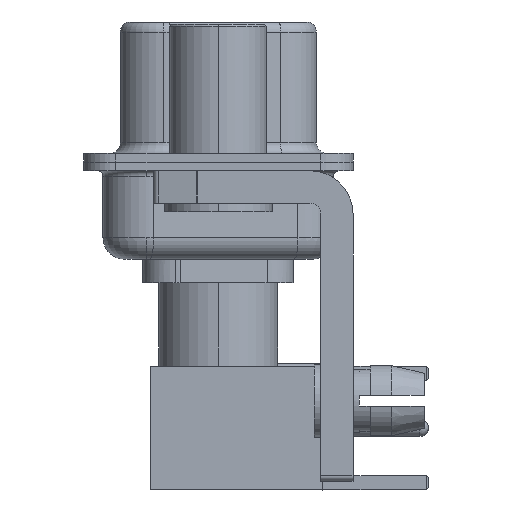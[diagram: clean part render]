
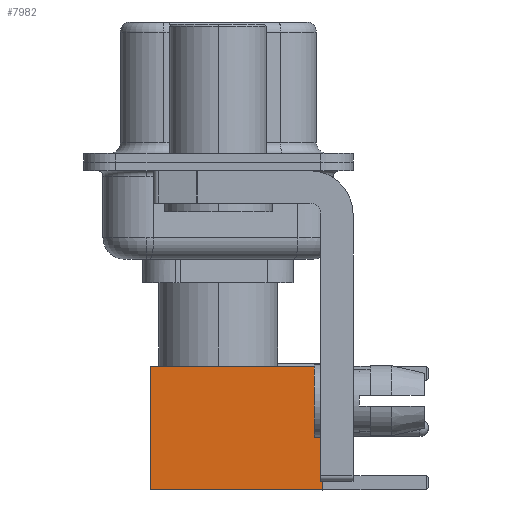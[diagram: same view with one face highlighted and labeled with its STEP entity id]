
A CAD part, left-side view. The second image highlights one B-rep face of the part: STEP entity #7982.
In plain terms, the highlighted face is planar.
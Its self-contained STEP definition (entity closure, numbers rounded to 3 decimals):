
#1560 = ORIENTED_EDGE ( 'NONE', *, *, #9778, .T. ) ;
#3294 = EDGE_CURVE ( 'NONE', #36083, #10672, #4469, .T. ) ;
#3545 = ORIENTED_EDGE ( 'NONE', *, *, #3294, .T. ) ;
#4402 = DIRECTION ( 'NONE',  ( 0., 0., -1. ) ) ;
#4469 = LINE ( 'NONE', #32501, #7651 ) ;
#4936 = VECTOR ( 'NONE', #4402, 1000. ) ;
#7360 = CARTESIAN_POINT ( 'NONE',  ( 2.875, 2.875, 0. ) ) ;
#7651 = VECTOR ( 'NONE', #9873, 1000. ) ;
#7982 = ADVANCED_FACE ( 'NONE', ( #8648 ), #34427, .T. ) ;
#8456 = AXIS2_PLACEMENT_3D ( 'NONE', #28863, #31286, #8818 ) ;
#8648 = FACE_OUTER_BOUND ( 'NONE', #25644, .T. ) ;
#8818 = DIRECTION ( 'NONE',  ( 0., 0., 1. ) ) ;
#9072 = DIRECTION ( 'NONE',  ( -1., 0., 0. ) ) ;
#9778 = EDGE_CURVE ( 'NONE', #26806, #36083, #9988, .T. ) ;
#9873 = DIRECTION ( 'NONE',  ( -1., 0., 0. ) ) ;
#9988 = LINE ( 'NONE', #16108, #4936 ) ;
#10267 = VECTOR ( 'NONE', #9072, 1000. ) ;
#10672 = VERTEX_POINT ( 'NONE', #14701 ) ;
#11019 = CARTESIAN_POINT ( 'NONE',  ( -2.875, 2.875, 8. ) ) ;
#11522 = LINE ( 'NONE', #22811, #10267 ) ;
#14701 = CARTESIAN_POINT ( 'NONE',  ( -2.875, 2.875, 0. ) ) ;
#15662 = VECTOR ( 'NONE', #23853, 1000. ) ;
#15912 = LINE ( 'NONE', #24601, #15662 ) ;
#16108 = CARTESIAN_POINT ( 'NONE',  ( 2.875, 2.875, 0. ) ) ;
#16491 = EDGE_CURVE ( 'NONE', #26806, #32471, #11522, .T. ) ;
#16589 = ORIENTED_EDGE ( 'NONE', *, *, #26795, .F. ) ;
#17587 = ORIENTED_EDGE ( 'NONE', *, *, #16491, .F. ) ;
#22811 = CARTESIAN_POINT ( 'NONE',  ( 0., 2.875, 8. ) ) ;
#23853 = DIRECTION ( 'NONE',  ( 0., 0., -1. ) ) ;
#24601 = CARTESIAN_POINT ( 'NONE',  ( -2.875, 2.875, 0. ) ) ;
#25644 = EDGE_LOOP ( 'NONE', ( #1560, #3545, #16589, #17587 ) ) ;
#26795 = EDGE_CURVE ( 'NONE', #32471, #10672, #15912, .T. ) ;
#26806 = VERTEX_POINT ( 'NONE', #27194 ) ;
#27194 = CARTESIAN_POINT ( 'NONE',  ( 2.875, 2.875, 8. ) ) ;
#28863 = CARTESIAN_POINT ( 'NONE',  ( 2.875, 2.875, 0. ) ) ;
#31286 = DIRECTION ( 'NONE',  ( 0., 1., 0. ) ) ;
#32471 = VERTEX_POINT ( 'NONE', #11019 ) ;
#32501 = CARTESIAN_POINT ( 'NONE',  ( 0., 2.875, 0. ) ) ;
#34427 = PLANE ( 'NONE',  #8456 ) ;
#36083 = VERTEX_POINT ( 'NONE', #7360 ) ;
